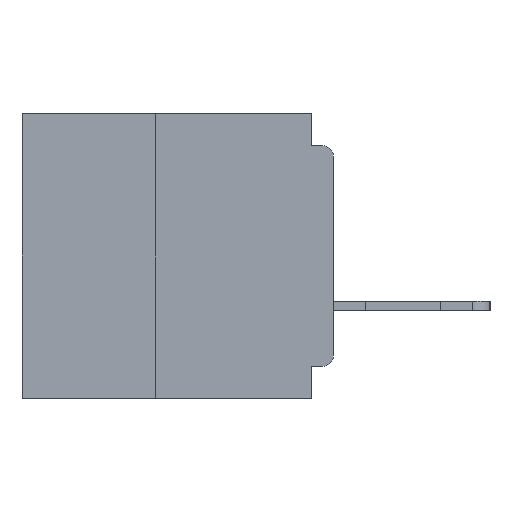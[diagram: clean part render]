
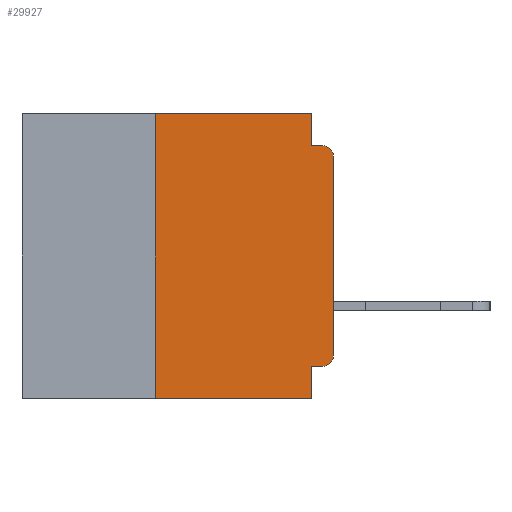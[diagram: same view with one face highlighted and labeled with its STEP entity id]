
A CAD part, left-side view. The second image highlights one B-rep face of the part: STEP entity #29927.
In plain terms, the highlighted planar face has unit normal (-1, 0, 0).
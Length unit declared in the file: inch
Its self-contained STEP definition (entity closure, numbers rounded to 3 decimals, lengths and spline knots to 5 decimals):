
#250 = EDGE_LOOP ( 'NONE', ( #12442, #34815, #56033, #35562, #19909, #44667, #22562, #35849, #40425, #12615 ) ) ;
#479 = DIRECTION ( 'NONE',  ( 0., 1., 0. ) ) ;
#2469 = EDGE_CURVE ( 'NONE', #54853, #53756, #43007, .T. ) ;
#2630 = LINE ( 'NONE', #17621, #23067 ) ;
#2697 = CARTESIAN_POINT ( 'NONE',  ( 0., 0.015, -0.34 ) ) ;
#4702 = VERTEX_POINT ( 'NONE', #52895 ) ;
#4753 = CARTESIAN_POINT ( 'NONE',  ( 0., 0.031, 0. ) ) ;
#4831 = VERTEX_POINT ( 'NONE', #14705 ) ;
#5866 = EDGE_CURVE ( 'NONE', #4831, #4702, #2630, .T. ) ;
#6771 = AXIS2_PLACEMENT_3D ( 'NONE', #19463, #19650, #49876 ) ;
#6978 = VECTOR ( 'NONE', #51846, 39.37008 ) ;
#7077 = DIRECTION ( 'NONE',  ( 0., 0., -1. ) ) ;
#7620 = CIRCLE ( 'NONE', #44974, 0.015 ) ;
#8260 = DIRECTION ( 'NONE',  ( -1., 0., 0. ) ) ;
#8395 = VECTOR ( 'NONE', #44394, 39.37008 ) ;
#9220 = VERTEX_POINT ( 'NONE', #44139 ) ;
#11276 = VECTOR ( 'NONE', #479, 39.37008 ) ;
#12442 = ORIENTED_EDGE ( 'NONE', *, *, #48873, .T. ) ;
#12615 = ORIENTED_EDGE ( 'NONE', *, *, #42204, .T. ) ;
#14705 = CARTESIAN_POINT ( 'NONE',  ( 0., 0.25, -0.4 ) ) ;
#14852 = CARTESIAN_POINT ( 'NONE',  ( 0., 0.015, -0.045 ) ) ;
#15303 = PLANE ( 'NONE',  #6771 ) ;
#17621 = CARTESIAN_POINT ( 'NONE',  ( 0., 0.25, -0.4 ) ) ;
#18486 = EDGE_CURVE ( 'NONE', #4702, #54853, #33241, .T. ) ;
#18588 = LINE ( 'NONE', #25964, #6978 ) ;
#19158 = VERTEX_POINT ( 'NONE', #23511 ) ;
#19463 = CARTESIAN_POINT ( 'NONE',  ( 0., 0.437, 0. ) ) ;
#19650 = DIRECTION ( 'NONE',  ( 1., 0., 0. ) ) ;
#19909 = ORIENTED_EDGE ( 'NONE', *, *, #18486, .F. ) ;
#20834 = CARTESIAN_POINT ( 'NONE',  ( 0., 0.031, -0.045 ) ) ;
#22562 = ORIENTED_EDGE ( 'NONE', *, *, #50988, .T. ) ;
#23067 = VECTOR ( 'NONE', #52184, 39.37008 ) ;
#23511 = CARTESIAN_POINT ( 'NONE',  ( 0., 0.031, -0.4 ) ) ;
#24384 = CARTESIAN_POINT ( 'NONE',  ( 0., 0., -0.045 ) ) ;
#24839 = FACE_OUTER_BOUND ( 'NONE', #250, .T. ) ;
#25800 = LINE ( 'NONE', #40679, #35921 ) ;
#25964 = CARTESIAN_POINT ( 'NONE',  ( 0., 0., 0. ) ) ;
#26236 = VECTOR ( 'NONE', #29204, 39.37008 ) ;
#26466 = CARTESIAN_POINT ( 'NONE',  ( 0., 0., -0.355 ) ) ;
#28683 = DIRECTION ( 'NONE',  ( 0., -1., 0. ) ) ;
#29204 = DIRECTION ( 'NONE',  ( 0., 0., -1. ) ) ;
#29927 = ADVANCED_FACE ( 'NONE', ( #24839 ), #15303, .F. ) ;
#31929 = CIRCLE ( 'NONE', #32674, 0.015 ) ;
#32674 = AXIS2_PLACEMENT_3D ( 'NONE', #34205, #8260, #38594 ) ;
#33036 = DIRECTION ( 'NONE',  ( -1., 0., 0. ) ) ;
#33153 = EDGE_CURVE ( 'NONE', #53632, #46571, #31929, .T. ) ;
#33241 = LINE ( 'NONE', #40385, #54915 ) ;
#34205 = CARTESIAN_POINT ( 'NONE',  ( 0., 0.015, -0.06 ) ) ;
#34815 = ORIENTED_EDGE ( 'NONE', *, *, #33153, .T. ) ;
#35562 = ORIENTED_EDGE ( 'NONE', *, *, #2469, .F. ) ;
#35849 = ORIENTED_EDGE ( 'NONE', *, *, #39909, .F. ) ;
#35921 = VECTOR ( 'NONE', #53722, 39.37008 ) ;
#36015 = DIRECTION ( 'NONE',  ( 0., -1., 0. ) ) ;
#38594 = DIRECTION ( 'NONE',  ( 0., 0., -1. ) ) ;
#39909 = EDGE_CURVE ( 'NONE', #49117, #19158, #46567, .T. ) ;
#40385 = CARTESIAN_POINT ( 'NONE',  ( 0., 0.437, 0. ) ) ;
#40425 = ORIENTED_EDGE ( 'NONE', *, *, #54214, .F. ) ;
#40679 = CARTESIAN_POINT ( 'NONE',  ( 0., 0.437, -0.4 ) ) ;
#41228 = CARTESIAN_POINT ( 'NONE',  ( 0., 0., -0.06 ) ) ;
#41363 = CARTESIAN_POINT ( 'NONE',  ( 0., 0.015, -0.355 ) ) ;
#42204 = EDGE_CURVE ( 'NONE', #44205, #9220, #7620, .T. ) ;
#42211 = EDGE_CURVE ( 'NONE', #53756, #46571, #42255, .T. ) ;
#42255 = LINE ( 'NONE', #24384, #52332 ) ;
#43007 = LINE ( 'NONE', #44761, #8395 ) ;
#44139 = CARTESIAN_POINT ( 'NONE',  ( 0., 0., -0.34 ) ) ;
#44205 = VERTEX_POINT ( 'NONE', #41363 ) ;
#44394 = DIRECTION ( 'NONE',  ( 0., 0., -1. ) ) ;
#44480 = LINE ( 'NONE', #26466, #11276 ) ;
#44667 = ORIENTED_EDGE ( 'NONE', *, *, #5866, .F. ) ;
#44761 = CARTESIAN_POINT ( 'NONE',  ( 0., 0.031, 0. ) ) ;
#44974 = AXIS2_PLACEMENT_3D ( 'NONE', #2697, #33036, #7077 ) ;
#46567 = LINE ( 'NONE', #55107, #26236 ) ;
#46571 = VERTEX_POINT ( 'NONE', #14852 ) ;
#48873 = EDGE_CURVE ( 'NONE', #9220, #53632, #18588, .T. ) ;
#49117 = VERTEX_POINT ( 'NONE', #53551 ) ;
#49876 = DIRECTION ( 'NONE',  ( 0., 0., -1. ) ) ;
#50988 = EDGE_CURVE ( 'NONE', #4831, #19158, #25800, .T. ) ;
#51846 = DIRECTION ( 'NONE',  ( 0., 0., 1. ) ) ;
#52184 = DIRECTION ( 'NONE',  ( 0., 0., 1. ) ) ;
#52332 = VECTOR ( 'NONE', #28683, 39.37008 ) ;
#52895 = CARTESIAN_POINT ( 'NONE',  ( 0., 0.25, 0. ) ) ;
#53551 = CARTESIAN_POINT ( 'NONE',  ( 0., 0.031, -0.355 ) ) ;
#53632 = VERTEX_POINT ( 'NONE', #41228 ) ;
#53722 = DIRECTION ( 'NONE',  ( 0., -1., 0. ) ) ;
#53756 = VERTEX_POINT ( 'NONE', #20834 ) ;
#54214 = EDGE_CURVE ( 'NONE', #44205, #49117, #44480, .T. ) ;
#54853 = VERTEX_POINT ( 'NONE', #4753 ) ;
#54915 = VECTOR ( 'NONE', #36015, 39.37008 ) ;
#55107 = CARTESIAN_POINT ( 'NONE',  ( 0., 0.031, -0.4 ) ) ;
#56033 = ORIENTED_EDGE ( 'NONE', *, *, #42211, .F. ) ;
